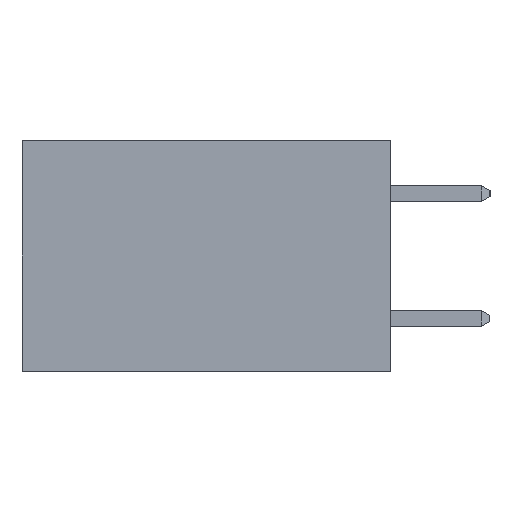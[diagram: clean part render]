
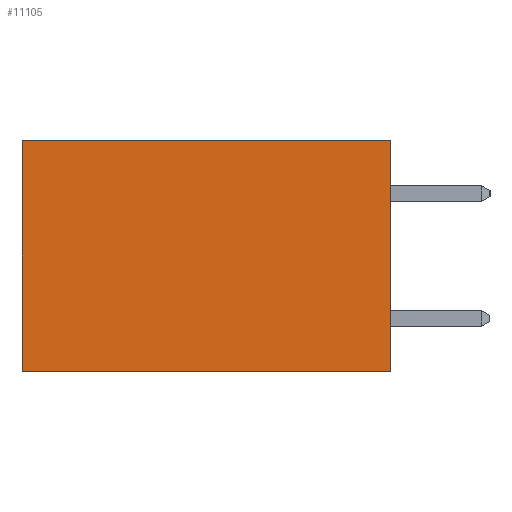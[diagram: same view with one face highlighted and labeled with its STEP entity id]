
A CAD part, left-side view. The second image highlights one B-rep face of the part: STEP entity #11105.
In plain terms, the highlighted planar face has unit normal (-1, 0, 0).
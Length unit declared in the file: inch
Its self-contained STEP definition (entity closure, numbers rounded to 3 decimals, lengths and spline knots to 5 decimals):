
#168 = VERTEX_POINT ( 'NONE', #12525 ) ;
#200 = CARTESIAN_POINT ( 'NONE',  ( 0.277, 0., -0.37 ) ) ;
#238 = DIRECTION ( 'NONE',  ( 0., 0., -1. ) ) ;
#354 = LINE ( 'NONE', #810, #8127 ) ;
#810 = CARTESIAN_POINT ( 'NONE',  ( 0.277, 0., -0.37 ) ) ;
#1571 = ORIENTED_EDGE ( 'NONE', *, *, #2989, .F. ) ;
#1989 = ORIENTED_EDGE ( 'NONE', *, *, #3848, .F. ) ;
#2047 = DIRECTION ( 'NONE',  ( 1., 0., 0. ) ) ;
#2101 = DIRECTION ( 'NONE',  ( 0., 1., 0. ) ) ;
#2989 = EDGE_CURVE ( 'NONE', #5400, #4496, #354, .T. ) ;
#3848 = EDGE_CURVE ( 'NONE', #168, #5400, #4533, .T. ) ;
#4496 = VERTEX_POINT ( 'NONE', #14065 ) ;
#4519 = PLANE ( 'NONE',  #9640 ) ;
#4533 = LINE ( 'NONE', #200, #13837 ) ;
#5283 = ORIENTED_EDGE ( 'NONE', *, *, #10224, .T. ) ;
#5400 = VERTEX_POINT ( 'NONE', #6215 ) ;
#5754 = CARTESIAN_POINT ( 'NONE',  ( 0.277, 0.59, -0.37 ) ) ;
#6215 = CARTESIAN_POINT ( 'NONE',  ( 0.277, 0., -0.37 ) ) ;
#6232 = LINE ( 'NONE', #5754, #15496 ) ;
#6563 = VECTOR ( 'NONE', #12743, 39.37008 ) ;
#6894 = CARTESIAN_POINT ( 'NONE',  ( 0.277, 0., -0.37 ) ) ;
#6939 = LINE ( 'NONE', #11540, #6563 ) ;
#7282 = FACE_OUTER_BOUND ( 'NONE', #14553, .T. ) ;
#8127 = VECTOR ( 'NONE', #2101, 39.37008 ) ;
#8188 = DIRECTION ( 'NONE',  ( 0., 0., -1. ) ) ;
#8881 = CARTESIAN_POINT ( 'NONE',  ( 0.277, 0.59, 0. ) ) ;
#9640 = AXIS2_PLACEMENT_3D ( 'NONE', #6894, #2047, #10650 ) ;
#10224 = EDGE_CURVE ( 'NONE', #168, #11388, #6939, .T. ) ;
#10650 = DIRECTION ( 'NONE',  ( 0., 0., -1. ) ) ;
#11040 = ORIENTED_EDGE ( 'NONE', *, *, #14351, .T. ) ;
#11105 = ADVANCED_FACE ( 'NONE', ( #7282 ), #4519, .F. ) ;
#11388 = VERTEX_POINT ( 'NONE', #8881 ) ;
#11540 = CARTESIAN_POINT ( 'NONE',  ( 0.277, 0., 0. ) ) ;
#12525 = CARTESIAN_POINT ( 'NONE',  ( 0.277, 0., 0. ) ) ;
#12743 = DIRECTION ( 'NONE',  ( 0., 1., 0. ) ) ;
#13837 = VECTOR ( 'NONE', #238, 39.37008 ) ;
#14065 = CARTESIAN_POINT ( 'NONE',  ( 0.277, 0.59, -0.37 ) ) ;
#14351 = EDGE_CURVE ( 'NONE', #11388, #4496, #6232, .T. ) ;
#14553 = EDGE_LOOP ( 'NONE', ( #11040, #1571, #1989, #5283 ) ) ;
#15496 = VECTOR ( 'NONE', #8188, 39.37008 ) ;
